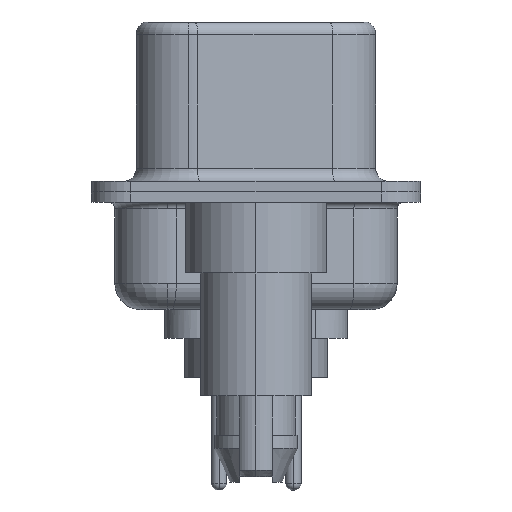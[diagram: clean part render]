
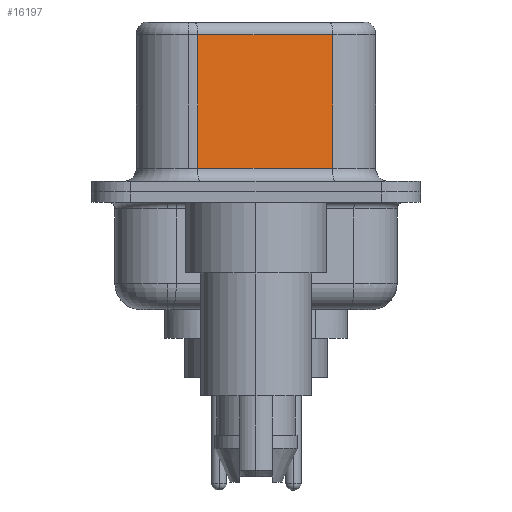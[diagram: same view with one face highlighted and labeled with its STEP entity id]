
A CAD part, left-side view. The second image highlights one B-rep face of the part: STEP entity #16197.
In plain terms, the highlighted planar face has unit normal (-0.985, -0.174, 0).
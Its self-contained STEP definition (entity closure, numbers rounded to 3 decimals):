
#778 = EDGE_CURVE ( 'NONE', #5914, #8932, #11656, .T. ) ;
#898 = EDGE_CURVE ( 'NONE', #5914, #19088, #11381, .T. ) ;
#948 = ORIENTED_EDGE ( 'NONE', *, *, #4078, .T. ) ;
#1147 = CARTESIAN_POINT ( 'NONE',  ( 4.585, -2.927, 6.02 ) ) ;
#2164 = ORIENTED_EDGE ( 'NONE', *, *, #17034, .T. ) ;
#2900 = FACE_OUTER_BOUND ( 'NONE', #13644, .T. ) ;
#4078 = EDGE_CURVE ( 'NONE', #19088, #14549, #5848, .T. ) ;
#4217 = DIRECTION ( 'NONE',  ( -0.174, 0.985, 0. ) ) ;
#4734 = VECTOR ( 'NONE', #11432, 1000. ) ;
#5848 = LINE ( 'NONE', #7208, #10294 ) ;
#5914 = VERTEX_POINT ( 'NONE', #16109 ) ;
#6934 = CARTESIAN_POINT ( 'NONE',  ( 3.675, 2.233, 6.02 ) ) ;
#6963 = CARTESIAN_POINT ( 'NONE',  ( 4.585, -2.927, 6.52 ) ) ;
#7194 = VECTOR ( 'NONE', #4217, 1000. ) ;
#7208 = CARTESIAN_POINT ( 'NONE',  ( 3.675, 2.233, 6.52 ) ) ;
#8932 = VERTEX_POINT ( 'NONE', #12461 ) ;
#8983 = DIRECTION ( 'NONE',  ( 0.985, 0.174, 0. ) ) ;
#10294 = VECTOR ( 'NONE', #12121, 1000. ) ;
#10779 = VECTOR ( 'NONE', #20145, 1000. ) ;
#11381 = LINE ( 'NONE', #1147, #7194 ) ;
#11432 = DIRECTION ( 'NONE',  ( 0., 0., -1. ) ) ;
#11656 = LINE ( 'NONE', #6963, #4734 ) ;
#12121 = DIRECTION ( 'NONE',  ( 0., 0., -1. ) ) ;
#12461 = CARTESIAN_POINT ( 'NONE',  ( 4.585, -2.927, 0.9 ) ) ;
#13644 = EDGE_LOOP ( 'NONE', ( #16404, #19284, #948, #2164 ) ) ;
#13978 = AXIS2_PLACEMENT_3D ( 'NONE', #18404, #8983, #20017 ) ;
#14549 = VERTEX_POINT ( 'NONE', #16194 ) ;
#14982 = LINE ( 'NONE', #15355, #10779 ) ;
#15355 = CARTESIAN_POINT ( 'NONE',  ( 4.585, -2.927, 0.9 ) ) ;
#16109 = CARTESIAN_POINT ( 'NONE',  ( 4.585, -2.927, 6.02 ) ) ;
#16194 = CARTESIAN_POINT ( 'NONE',  ( 3.675, 2.233, 0.9 ) ) ;
#16197 = ADVANCED_FACE ( 'NONE', ( #2900 ), #16824, .F. ) ;
#16404 = ORIENTED_EDGE ( 'NONE', *, *, #778, .F. ) ;
#16824 = PLANE ( 'NONE',  #13978 ) ;
#17034 = EDGE_CURVE ( 'NONE', #14549, #8932, #14982, .T. ) ;
#18404 = CARTESIAN_POINT ( 'NONE',  ( 4.585, -2.927, 6.52 ) ) ;
#19088 = VERTEX_POINT ( 'NONE', #6934 ) ;
#19284 = ORIENTED_EDGE ( 'NONE', *, *, #898, .T. ) ;
#20017 = DIRECTION ( 'NONE',  ( -0.174, 0.985, 0. ) ) ;
#20145 = DIRECTION ( 'NONE',  ( 0.174, -0.985, 0. ) ) ;
